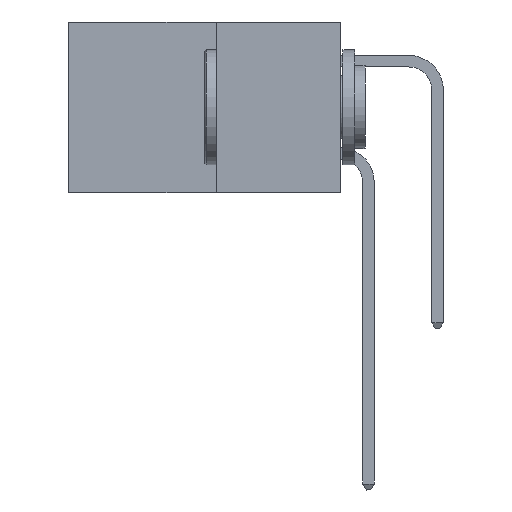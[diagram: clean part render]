
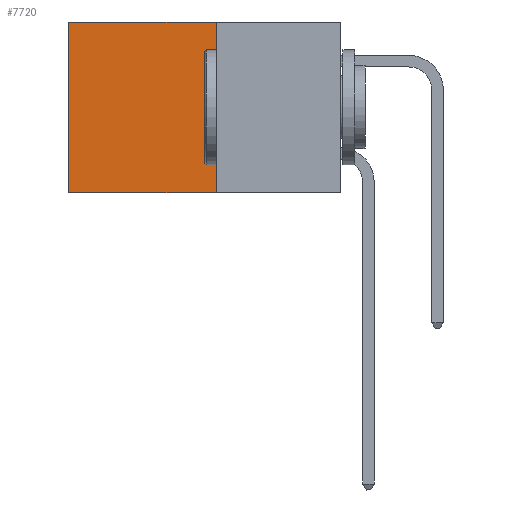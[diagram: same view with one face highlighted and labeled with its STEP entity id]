
A CAD part, left-side view. The second image highlights one B-rep face of the part: STEP entity #7720.
In plain terms, the highlighted planar face has unit normal (-1, 0, 0).
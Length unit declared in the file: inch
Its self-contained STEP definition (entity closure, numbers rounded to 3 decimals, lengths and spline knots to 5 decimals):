
#171 = LINE ( 'NONE', #6226, #9436 ) ;
#244 = LINE ( 'NONE', #8677, #3043 ) ;
#1039 = DIRECTION ( 'NONE',  ( 0., 0., -1. ) ) ;
#1043 = CARTESIAN_POINT ( 'NONE',  ( 0.277, 0.27, -0.37 ) ) ;
#1448 = LINE ( 'NONE', #13757, #4320 ) ;
#2380 = VECTOR ( 'NONE', #1039, 39.37008 ) ;
#2677 = ORIENTED_EDGE ( 'NONE', *, *, #7249, .T. ) ;
#2934 = DIRECTION ( 'NONE',  ( 0., 0., -1. ) ) ;
#2955 = DIRECTION ( 'NONE',  ( 1., 0., 0. ) ) ;
#2986 = PLANE ( 'NONE',  #6495 ) ;
#2991 = CARTESIAN_POINT ( 'NONE',  ( 0.277, 0.27, -0.37 ) ) ;
#3043 = VECTOR ( 'NONE', #7090, 39.37008 ) ;
#3093 = VERTEX_POINT ( 'NONE', #14303 ) ;
#3125 = CARTESIAN_POINT ( 'NONE',  ( 0.277, 0.59, 0. ) ) ;
#4176 = CARTESIAN_POINT ( 'NONE',  ( 0.277, 0.59, -0.37 ) ) ;
#4256 = EDGE_CURVE ( 'NONE', #14627, #10040, #244, .T. ) ;
#4320 = VECTOR ( 'NONE', #13669, 39.37008 ) ;
#5210 = ORIENTED_EDGE ( 'NONE', *, *, #7995, .F. ) ;
#5686 = ORIENTED_EDGE ( 'NONE', *, *, #4256, .F. ) ;
#6143 = ORIENTED_EDGE ( 'NONE', *, *, #6213, .T. ) ;
#6163 = DIRECTION ( 'NONE',  ( 0., 1., 0. ) ) ;
#6198 = FACE_OUTER_BOUND ( 'NONE', #9872, .T. ) ;
#6213 = EDGE_CURVE ( 'NONE', #7723, #10040, #1448, .T. ) ;
#6226 = CARTESIAN_POINT ( 'NONE',  ( 0.277, 0.27, 0. ) ) ;
#6495 = AXIS2_PLACEMENT_3D ( 'NONE', #2991, #2955, #2934 ) ;
#7090 = DIRECTION ( 'NONE',  ( 0., 1., 0. ) ) ;
#7249 = EDGE_CURVE ( 'NONE', #3093, #7723, #171, .T. ) ;
#7720 = ADVANCED_FACE ( 'NONE', ( #6198 ), #2986, .F. ) ;
#7723 = VERTEX_POINT ( 'NONE', #3125 ) ;
#7995 = EDGE_CURVE ( 'NONE', #3093, #14627, #14755, .T. ) ;
#8677 = CARTESIAN_POINT ( 'NONE',  ( 0.277, 0.27, -0.37 ) ) ;
#9436 = VECTOR ( 'NONE', #6163, 39.37008 ) ;
#9872 = EDGE_LOOP ( 'NONE', ( #6143, #5686, #5210, #2677 ) ) ;
#10040 = VERTEX_POINT ( 'NONE', #4176 ) ;
#12052 = CARTESIAN_POINT ( 'NONE',  ( 0.277, 0.27, -0.37 ) ) ;
#13669 = DIRECTION ( 'NONE',  ( 0., 0., -1. ) ) ;
#13757 = CARTESIAN_POINT ( 'NONE',  ( 0.277, 0.59, -0.37 ) ) ;
#14303 = CARTESIAN_POINT ( 'NONE',  ( 0.277, 0.27, 0. ) ) ;
#14627 = VERTEX_POINT ( 'NONE', #12052 ) ;
#14755 = LINE ( 'NONE', #1043, #2380 ) ;
